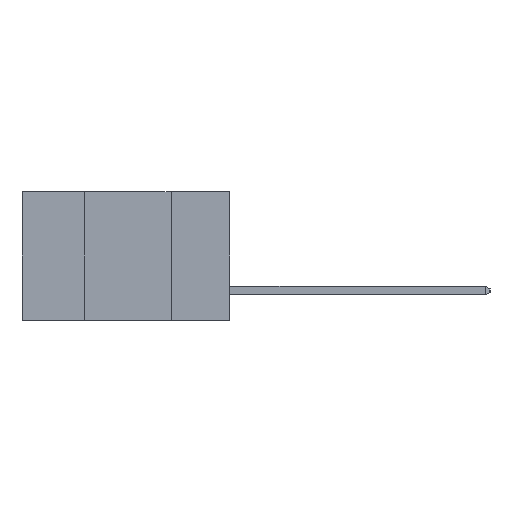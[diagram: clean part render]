
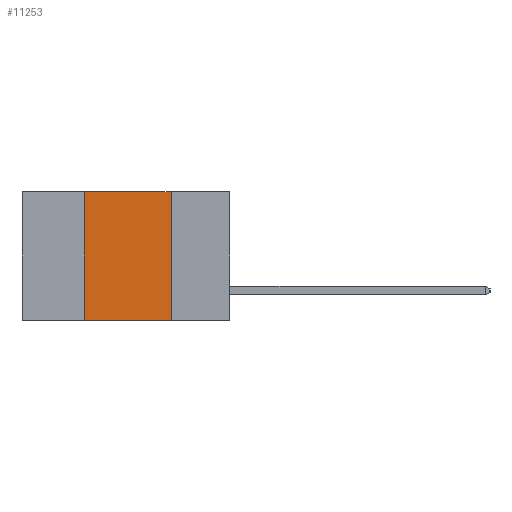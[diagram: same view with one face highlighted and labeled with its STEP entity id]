
A CAD part, left-side view. The second image highlights one B-rep face of the part: STEP entity #11253.
In plain terms, the highlighted planar face has unit normal (-1, 0, 0).
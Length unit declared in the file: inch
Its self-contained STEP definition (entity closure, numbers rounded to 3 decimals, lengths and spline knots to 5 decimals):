
#6 = EDGE_CURVE ( 'NONE', #3525, #5831, #9849, .T. ) ;
#66 = ORIENTED_EDGE ( 'NONE', *, *, #7006, .F. ) ;
#163 = LINE ( 'NONE', #9030, #11783 ) ;
#613 = DIRECTION ( 'NONE',  ( 1., 0., 0. ) ) ;
#1632 = DIRECTION ( 'NONE',  ( 0., 0., -1. ) ) ;
#1709 = CARTESIAN_POINT ( 'NONE',  ( 0., 0.17, 0. ) ) ;
#1875 = VECTOR ( 'NONE', #4719, 39.37008 ) ;
#2612 = VERTEX_POINT ( 'NONE', #3117 ) ;
#2657 = EDGE_CURVE ( 'NONE', #3525, #2612, #4342, .T. ) ;
#2837 = ORIENTED_EDGE ( 'NONE', *, *, #2657, .T. ) ;
#3117 = CARTESIAN_POINT ( 'NONE',  ( 0., 0.17, -0.37 ) ) ;
#3158 = DIRECTION ( 'NONE',  ( 0., -1., 0. ) ) ;
#3525 = VERTEX_POINT ( 'NONE', #8169 ) ;
#3970 = ORIENTED_EDGE ( 'NONE', *, *, #6, .F. ) ;
#4342 = LINE ( 'NONE', #9490, #11673 ) ;
#4719 = DIRECTION ( 'NONE',  ( 0., -1., 0. ) ) ;
#4766 = ORIENTED_EDGE ( 'NONE', *, *, #7372, .F. ) ;
#4874 = CARTESIAN_POINT ( 'NONE',  ( 0., 0.42, 0. ) ) ;
#5406 = PLANE ( 'NONE',  #8322 ) ;
#5430 = DIRECTION ( 'NONE',  ( 0., 0., 1. ) ) ;
#5831 = VERTEX_POINT ( 'NONE', #4874 ) ;
#6159 = FACE_OUTER_BOUND ( 'NONE', #9145, .T. ) ;
#6578 = CARTESIAN_POINT ( 'NONE',  ( 0., 0.6, 0. ) ) ;
#7006 = EDGE_CURVE ( 'NONE', #5831, #11321, #9232, .T. ) ;
#7251 = DIRECTION ( 'NONE',  ( 0., 0., -1. ) ) ;
#7372 = EDGE_CURVE ( 'NONE', #11321, #2612, #163, .T. ) ;
#7525 = VECTOR ( 'NONE', #5430, 39.37008 ) ;
#7827 = CARTESIAN_POINT ( 'NONE',  ( 0., 0.42, -0.37 ) ) ;
#8169 = CARTESIAN_POINT ( 'NONE',  ( 0., 0.42, -0.37 ) ) ;
#8322 = AXIS2_PLACEMENT_3D ( 'NONE', #9853, #613, #7251 ) ;
#9030 = CARTESIAN_POINT ( 'NONE',  ( 0., 0.17, -0.37 ) ) ;
#9145 = EDGE_LOOP ( 'NONE', ( #4766, #66, #3970, #2837 ) ) ;
#9232 = LINE ( 'NONE', #6578, #1875 ) ;
#9490 = CARTESIAN_POINT ( 'NONE',  ( 0., 0.6, -0.37 ) ) ;
#9849 = LINE ( 'NONE', #7827, #7525 ) ;
#9853 = CARTESIAN_POINT ( 'NONE',  ( 0., 0.6, 0. ) ) ;
#11253 = ADVANCED_FACE ( 'NONE', ( #6159 ), #5406, .F. ) ;
#11321 = VERTEX_POINT ( 'NONE', #1709 ) ;
#11673 = VECTOR ( 'NONE', #3158, 39.37008 ) ;
#11783 = VECTOR ( 'NONE', #1632, 39.37008 ) ;
